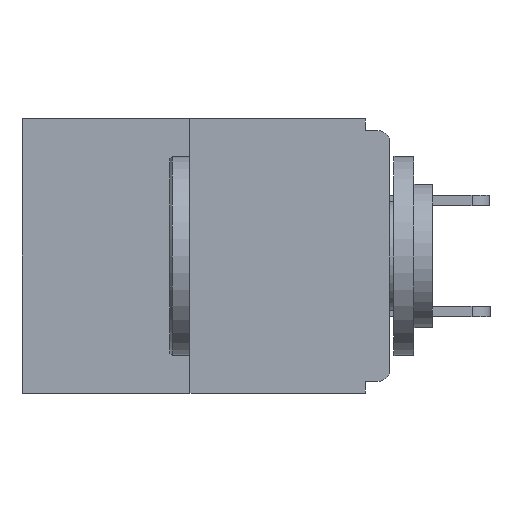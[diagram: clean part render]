
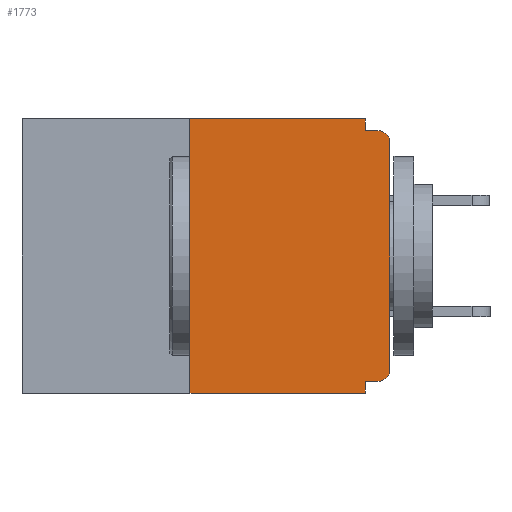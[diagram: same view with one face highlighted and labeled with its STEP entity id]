
A CAD part, left-side view. The second image highlights one B-rep face of the part: STEP entity #1773.
In plain terms, the highlighted planar face has unit normal (-1, 0, 0).
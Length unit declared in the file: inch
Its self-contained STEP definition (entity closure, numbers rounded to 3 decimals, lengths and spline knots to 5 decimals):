
#216 = PLANE ( 'NONE',  #24341 ) ;
#648 = DIRECTION ( 'NONE',  ( -1., 0., 0. ) ) ;
#873 = VERTEX_POINT ( 'NONE', #31560 ) ;
#1773 = ADVANCED_FACE ( 'NONE', ( #19557 ), #216, .F. ) ;
#1875 = LINE ( 'NONE', #14218, #15353 ) ;
#2477 = VERTEX_POINT ( 'NONE', #31576 ) ;
#2957 = VECTOR ( 'NONE', #31680, 39.37008 ) ;
#3630 = EDGE_CURVE ( 'NONE', #20276, #9565, #24126, .T. ) ;
#3653 = VECTOR ( 'NONE', #24453, 39.37008 ) ;
#4550 = DIRECTION ( 'NONE',  ( 0., 0., -1. ) ) ;
#5283 = VECTOR ( 'NONE', #5943, 39.37008 ) ;
#5299 = CARTESIAN_POINT ( 'NONE',  ( 0., 0.015, -0.03 ) ) ;
#5330 = VERTEX_POINT ( 'NONE', #12817 ) ;
#5376 = DIRECTION ( 'NONE',  ( 0., 1., 0. ) ) ;
#5655 = EDGE_CURVE ( 'NONE', #2477, #9760, #19650, .T. ) ;
#5907 = EDGE_CURVE ( 'NONE', #5330, #873, #10018, .T. ) ;
#5943 = DIRECTION ( 'NONE',  ( 0., 0., 1. ) ) ;
#6057 = EDGE_CURVE ( 'NONE', #8567, #2477, #7287, .T. ) ;
#6113 = ORIENTED_EDGE ( 'NONE', *, *, #5655, .F. ) ;
#6437 = EDGE_CURVE ( 'NONE', #20276, #30403, #22658, .T. ) ;
#7287 = LINE ( 'NONE', #18108, #15726 ) ;
#7697 = DIRECTION ( 'NONE',  ( 0., 0., -1. ) ) ;
#8567 = VERTEX_POINT ( 'NONE', #30876 ) ;
#9226 = ORIENTED_EDGE ( 'NONE', *, *, #16745, .T. ) ;
#9548 = CARTESIAN_POINT ( 'NONE',  ( 0., 0., -0.328 ) ) ;
#9565 = VERTEX_POINT ( 'NONE', #15209 ) ;
#9760 = VERTEX_POINT ( 'NONE', #16503 ) ;
#10018 = LINE ( 'NONE', #9548, #21940 ) ;
#10098 = CARTESIAN_POINT ( 'NONE',  ( 0., 0.46, 0. ) ) ;
#10185 = AXIS2_PLACEMENT_3D ( 'NONE', #12735, #648, #20381 ) ;
#10868 = VERTEX_POINT ( 'NONE', #12693 ) ;
#11779 = CARTESIAN_POINT ( 'NONE',  ( 0., 0.46, -0.343 ) ) ;
#12693 = CARTESIAN_POINT ( 'NONE',  ( 0., 0., -0.03 ) ) ;
#12735 = CARTESIAN_POINT ( 'NONE',  ( 0., 0.015, -0.313 ) ) ;
#12743 = DIRECTION ( 'NONE',  ( -1., 0., 0. ) ) ;
#12817 = CARTESIAN_POINT ( 'NONE',  ( 0., 0.015, -0.328 ) ) ;
#12837 = DIRECTION ( 'NONE',  ( 1., 0., 0. ) ) ;
#12905 = CARTESIAN_POINT ( 'NONE',  ( 0., 0.46, 0. ) ) ;
#14218 = CARTESIAN_POINT ( 'NONE',  ( 0., 0.031, -0.343 ) ) ;
#15111 = ORIENTED_EDGE ( 'NONE', *, *, #6437, .F. ) ;
#15167 = DIRECTION ( 'NONE',  ( 0., -1., 0. ) ) ;
#15209 = CARTESIAN_POINT ( 'NONE',  ( 0., 0.031, -0.343 ) ) ;
#15353 = VECTOR ( 'NONE', #21640, 39.37008 ) ;
#15386 = ORIENTED_EDGE ( 'NONE', *, *, #5907, .F. ) ;
#15589 = DIRECTION ( 'NONE',  ( 0., 0., -1. ) ) ;
#15726 = VECTOR ( 'NONE', #15589, 39.37008 ) ;
#16445 = LINE ( 'NONE', #26735, #2957 ) ;
#16451 = EDGE_CURVE ( 'NONE', #30403, #8567, #29293, .T. ) ;
#16503 = CARTESIAN_POINT ( 'NONE',  ( 0., 0.015, -0.015 ) ) ;
#16617 = DIRECTION ( 'NONE',  ( 0., -1., 0. ) ) ;
#16745 = EDGE_CURVE ( 'NONE', #5330, #27497, #23450, .T. ) ;
#16765 = ORIENTED_EDGE ( 'NONE', *, *, #28044, .F. ) ;
#17458 = EDGE_CURVE ( 'NONE', #27497, #10868, #16445, .T. ) ;
#18108 = CARTESIAN_POINT ( 'NONE',  ( 0., 0.031, 0. ) ) ;
#18398 = CARTESIAN_POINT ( 'NONE',  ( 0., 0.25, 0. ) ) ;
#18492 = CARTESIAN_POINT ( 'NONE',  ( 0., 0.25, 0. ) ) ;
#18855 = VECTOR ( 'NONE', #15167, 39.37008 ) ;
#18899 = ORIENTED_EDGE ( 'NONE', *, *, #6057, .F. ) ;
#19557 = FACE_OUTER_BOUND ( 'NONE', #23957, .T. ) ;
#19618 = CARTESIAN_POINT ( 'NONE',  ( 0., 0., -0.313 ) ) ;
#19650 = LINE ( 'NONE', #20816, #27381 ) ;
#20276 = VERTEX_POINT ( 'NONE', #28453 ) ;
#20381 = DIRECTION ( 'NONE',  ( 0., 0., -1. ) ) ;
#20816 = CARTESIAN_POINT ( 'NONE',  ( 0., 0., -0.015 ) ) ;
#21258 = ORIENTED_EDGE ( 'NONE', *, *, #17458, .T. ) ;
#21640 = DIRECTION ( 'NONE',  ( 0., 0., -1. ) ) ;
#21861 = ORIENTED_EDGE ( 'NONE', *, *, #3630, .T. ) ;
#21940 = VECTOR ( 'NONE', #5376, 39.37008 ) ;
#22658 = LINE ( 'NONE', #18492, #5283 ) ;
#23450 = CIRCLE ( 'NONE', #10185, 0.015 ) ;
#23957 = EDGE_LOOP ( 'NONE', ( #31015, #15111, #21861, #16765, #15386, #9226, #21258, #31284, #6113, #18899 ) ) ;
#24115 = CIRCLE ( 'NONE', #31275, 0.015 ) ;
#24126 = LINE ( 'NONE', #11779, #3653 ) ;
#24341 = AXIS2_PLACEMENT_3D ( 'NONE', #10098, #12837, #7697 ) ;
#24453 = DIRECTION ( 'NONE',  ( 0., -1., 0. ) ) ;
#26735 = CARTESIAN_POINT ( 'NONE',  ( 0., 0., 0. ) ) ;
#27381 = VECTOR ( 'NONE', #16617, 39.37008 ) ;
#27497 = VERTEX_POINT ( 'NONE', #19618 ) ;
#28044 = EDGE_CURVE ( 'NONE', #873, #9565, #1875, .T. ) ;
#28453 = CARTESIAN_POINT ( 'NONE',  ( 0., 0.25, -0.343 ) ) ;
#29293 = LINE ( 'NONE', #12905, #18855 ) ;
#30403 = VERTEX_POINT ( 'NONE', #18398 ) ;
#30729 = EDGE_CURVE ( 'NONE', #10868, #9760, #24115, .T. ) ;
#30876 = CARTESIAN_POINT ( 'NONE',  ( 0., 0.031, 0. ) ) ;
#31015 = ORIENTED_EDGE ( 'NONE', *, *, #16451, .F. ) ;
#31275 = AXIS2_PLACEMENT_3D ( 'NONE', #5299, #12743, #4550 ) ;
#31284 = ORIENTED_EDGE ( 'NONE', *, *, #30729, .T. ) ;
#31560 = CARTESIAN_POINT ( 'NONE',  ( 0., 0.031, -0.328 ) ) ;
#31576 = CARTESIAN_POINT ( 'NONE',  ( 0., 0.031, -0.015 ) ) ;
#31680 = DIRECTION ( 'NONE',  ( 0., 0., 1. ) ) ;
